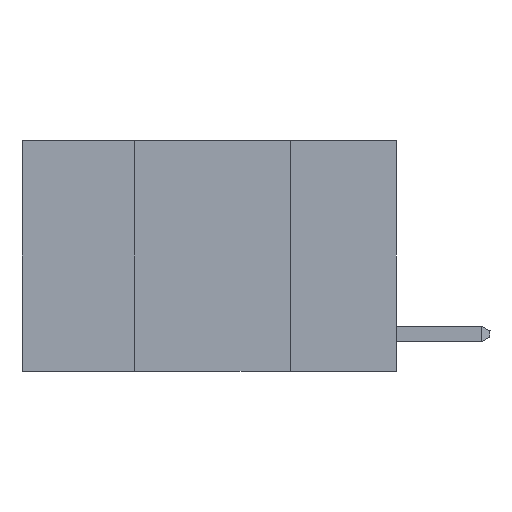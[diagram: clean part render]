
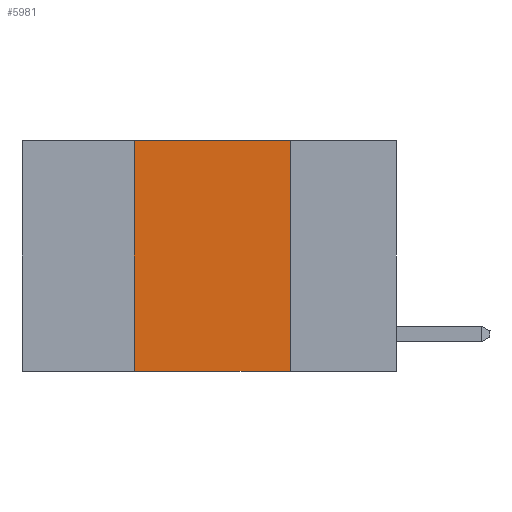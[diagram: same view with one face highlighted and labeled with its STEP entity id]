
A CAD part, left-side view. The second image highlights one B-rep face of the part: STEP entity #5981.
In plain terms, the highlighted planar face has unit normal (-1, 0, 0).
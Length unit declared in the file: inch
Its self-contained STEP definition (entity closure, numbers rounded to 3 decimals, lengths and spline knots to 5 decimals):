
#114 = CARTESIAN_POINT ( 'NONE',  ( 0., 0.6, 0. ) ) ;
#344 = EDGE_CURVE ( 'NONE', #9525, #8276, #10876, .T. ) ;
#1521 = LINE ( 'NONE', #5537, #10273 ) ;
#1896 = CARTESIAN_POINT ( 'NONE',  ( 0., 0.42, 0. ) ) ;
#2560 = AXIS2_PLACEMENT_3D ( 'NONE', #114, #10099, #6485 ) ;
#3778 = DIRECTION ( 'NONE',  ( 0., 0., -1. ) ) ;
#3805 = LINE ( 'NONE', #3901, #11689 ) ;
#3901 = CARTESIAN_POINT ( 'NONE',  ( 0., 0.42, 0. ) ) ;
#4673 = LINE ( 'NONE', #7574, #8247 ) ;
#5195 = CARTESIAN_POINT ( 'NONE',  ( 0., 0.42, -0.37 ) ) ;
#5283 = CARTESIAN_POINT ( 'NONE',  ( 0., 0.17, 0. ) ) ;
#5308 = VERTEX_POINT ( 'NONE', #5195 ) ;
#5537 = CARTESIAN_POINT ( 'NONE',  ( 0., 0.6, -0.37 ) ) ;
#5962 = VERTEX_POINT ( 'NONE', #1896 ) ;
#5981 = ADVANCED_FACE ( 'NONE', ( #11441 ), #9103, .F. ) ;
#6272 = CARTESIAN_POINT ( 'NONE',  ( 0., 0.17, -0.37 ) ) ;
#6485 = DIRECTION ( 'NONE',  ( 0., 0., -1. ) ) ;
#7439 = DIRECTION ( 'NONE',  ( 0., -1., 0. ) ) ;
#7546 = DIRECTION ( 'NONE',  ( 0., 0., 1. ) ) ;
#7574 = CARTESIAN_POINT ( 'NONE',  ( 0., 0.6, 0. ) ) ;
#7653 = DIRECTION ( 'NONE',  ( 0., -1., 0. ) ) ;
#8141 = ORIENTED_EDGE ( 'NONE', *, *, #10463, .F. ) ;
#8234 = ORIENTED_EDGE ( 'NONE', *, *, #9707, .T. ) ;
#8247 = VECTOR ( 'NONE', #7653, 39.37008 ) ;
#8276 = VERTEX_POINT ( 'NONE', #6272 ) ;
#8438 = EDGE_LOOP ( 'NONE', ( #11242, #8141, #11736, #8234 ) ) ;
#9103 = PLANE ( 'NONE',  #2560 ) ;
#9235 = CARTESIAN_POINT ( 'NONE',  ( 0., 0.17, 0. ) ) ;
#9525 = VERTEX_POINT ( 'NONE', #5283 ) ;
#9707 = EDGE_CURVE ( 'NONE', #5308, #8276, #1521, .T. ) ;
#10099 = DIRECTION ( 'NONE',  ( 1., 0., 0. ) ) ;
#10273 = VECTOR ( 'NONE', #7439, 39.37008 ) ;
#10463 = EDGE_CURVE ( 'NONE', #5962, #9525, #4673, .T. ) ;
#10498 = EDGE_CURVE ( 'NONE', #5308, #5962, #3805, .T. ) ;
#10876 = LINE ( 'NONE', #9235, #11184 ) ;
#11184 = VECTOR ( 'NONE', #3778, 39.37008 ) ;
#11242 = ORIENTED_EDGE ( 'NONE', *, *, #344, .F. ) ;
#11441 = FACE_OUTER_BOUND ( 'NONE', #8438, .T. ) ;
#11689 = VECTOR ( 'NONE', #7546, 39.37008 ) ;
#11736 = ORIENTED_EDGE ( 'NONE', *, *, #10498, .F. ) ;
